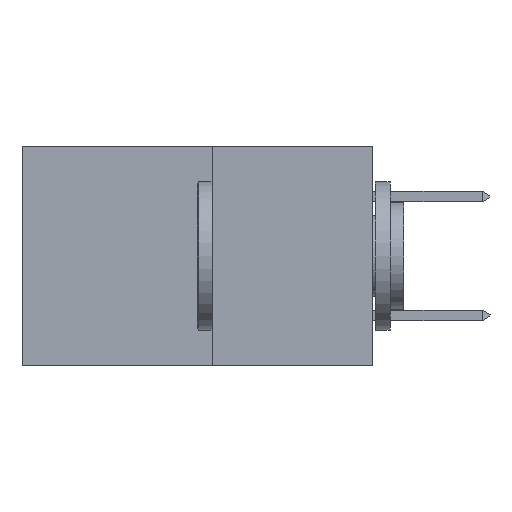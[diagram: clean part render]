
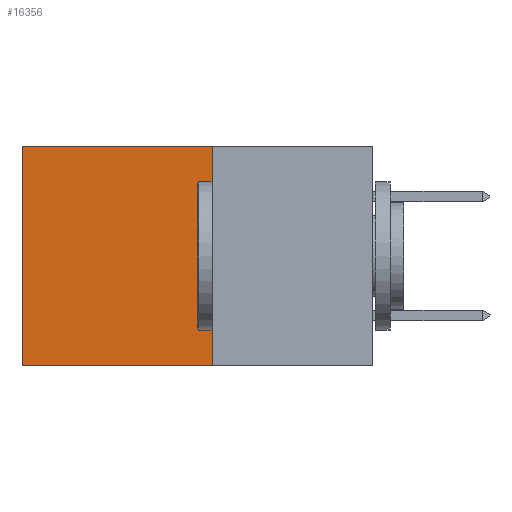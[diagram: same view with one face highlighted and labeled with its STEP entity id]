
A CAD part, left-side view. The second image highlights one B-rep face of the part: STEP entity #16356.
In plain terms, the highlighted planar face has unit normal (-1, 0, 0).
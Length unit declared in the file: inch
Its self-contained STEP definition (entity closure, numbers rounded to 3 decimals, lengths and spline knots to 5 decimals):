
#2118 = LINE ( 'NONE', #23525, #8359 ) ;
#4427 = FACE_OUTER_BOUND ( 'NONE', #31895, .T. ) ;
#4985 = DIRECTION ( 'NONE',  ( 0., 1., 0. ) ) ;
#8359 = VECTOR ( 'NONE', #31292, 39.37008 ) ;
#9932 = PLANE ( 'NONE',  #14788 ) ;
#10333 = VERTEX_POINT ( 'NONE', #26668 ) ;
#10484 = EDGE_CURVE ( 'NONE', #14717, #10333, #23853, .T. ) ;
#10747 = VECTOR ( 'NONE', #4985, 39.37008 ) ;
#11080 = ORIENTED_EDGE ( 'NONE', *, *, #26842, .F. ) ;
#11203 = DIRECTION ( 'NONE',  ( 0., 0., -1. ) ) ;
#11607 = VECTOR ( 'NONE', #27296, 39.37008 ) ;
#14127 = CARTESIAN_POINT ( 'NONE',  ( 0.277, 0.27, -0.37 ) ) ;
#14717 = VERTEX_POINT ( 'NONE', #29882 ) ;
#14788 = AXIS2_PLACEMENT_3D ( 'NONE', #22995, #30780, #15231 ) ;
#15124 = ORIENTED_EDGE ( 'NONE', *, *, #10484, .T. ) ;
#15231 = DIRECTION ( 'NONE',  ( 0., 0., -1. ) ) ;
#16356 = ADVANCED_FACE ( 'NONE', ( #4427 ), #9932, .F. ) ;
#18564 = LINE ( 'NONE', #14127, #11607 ) ;
#19294 = VECTOR ( 'NONE', #11203, 39.37008 ) ;
#22995 = CARTESIAN_POINT ( 'NONE',  ( 0.277, 0.27, -0.37 ) ) ;
#22999 = VERTEX_POINT ( 'NONE', #32893 ) ;
#23433 = VERTEX_POINT ( 'NONE', #26545 ) ;
#23525 = CARTESIAN_POINT ( 'NONE',  ( 0.277, 0.59, -0.37 ) ) ;
#23853 = LINE ( 'NONE', #29557, #10747 ) ;
#24273 = CARTESIAN_POINT ( 'NONE',  ( 0.277, 0.27, -0.37 ) ) ;
#26077 = EDGE_CURVE ( 'NONE', #10333, #23433, #2118, .T. ) ;
#26545 = CARTESIAN_POINT ( 'NONE',  ( 0.277, 0.59, -0.37 ) ) ;
#26668 = CARTESIAN_POINT ( 'NONE',  ( 0.277, 0.59, 0. ) ) ;
#26842 = EDGE_CURVE ( 'NONE', #22999, #23433, #18564, .T. ) ;
#27296 = DIRECTION ( 'NONE',  ( 0., 1., 0. ) ) ;
#29557 = CARTESIAN_POINT ( 'NONE',  ( 0.277, 0.27, 0. ) ) ;
#29882 = CARTESIAN_POINT ( 'NONE',  ( 0.277, 0.27, 0. ) ) ;
#29973 = ORIENTED_EDGE ( 'NONE', *, *, #32410, .F. ) ;
#30780 = DIRECTION ( 'NONE',  ( 1., 0., 0. ) ) ;
#31292 = DIRECTION ( 'NONE',  ( 0., 0., -1. ) ) ;
#31895 = EDGE_LOOP ( 'NONE', ( #33562, #11080, #29973, #15124 ) ) ;
#32410 = EDGE_CURVE ( 'NONE', #14717, #22999, #33832, .T. ) ;
#32893 = CARTESIAN_POINT ( 'NONE',  ( 0.277, 0.27, -0.37 ) ) ;
#33562 = ORIENTED_EDGE ( 'NONE', *, *, #26077, .T. ) ;
#33832 = LINE ( 'NONE', #24273, #19294 ) ;
